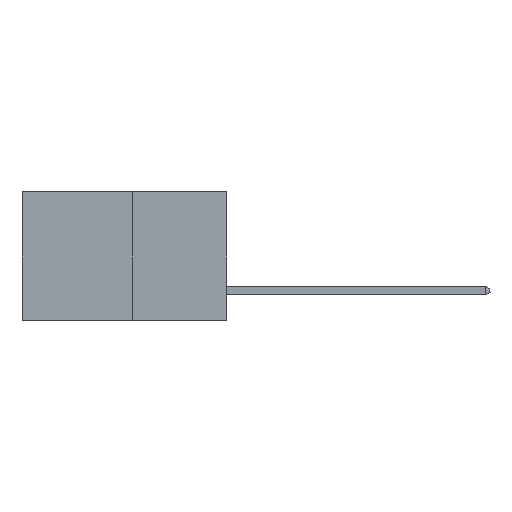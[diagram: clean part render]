
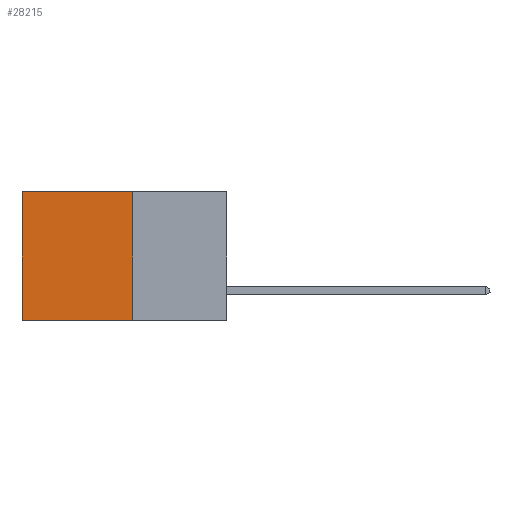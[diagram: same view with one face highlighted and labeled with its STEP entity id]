
A CAD part, left-side view. The second image highlights one B-rep face of the part: STEP entity #28215.
In plain terms, the highlighted planar face has unit normal (-1, 0, 0).
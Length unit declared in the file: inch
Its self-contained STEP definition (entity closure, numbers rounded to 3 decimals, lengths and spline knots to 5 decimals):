
#1632 = DIRECTION ( 'NONE',  ( 0., 0., -1. ) ) ;
#1753 = CARTESIAN_POINT ( 'NONE',  ( 0.277, 0.27, -0.37 ) ) ;
#2047 = AXIS2_PLACEMENT_3D ( 'NONE', #32463, #16976, #1632 ) ;
#2958 = ORIENTED_EDGE ( 'NONE', *, *, #8864, .T. ) ;
#3737 = FACE_OUTER_BOUND ( 'NONE', #17439, .T. ) ;
#4024 = VERTEX_POINT ( 'NONE', #24812 ) ;
#4605 = DIRECTION ( 'NONE',  ( 0., 1., 0. ) ) ;
#6934 = DIRECTION ( 'NONE',  ( 0., 0., -1. ) ) ;
#8864 = EDGE_CURVE ( 'NONE', #4024, #20282, #24092, .T. ) ;
#10590 = VECTOR ( 'NONE', #4605, 39.37008 ) ;
#11789 = EDGE_CURVE ( 'NONE', #11993, #17563, #14049, .T. ) ;
#11973 = ORIENTED_EDGE ( 'NONE', *, *, #11789, .F. ) ;
#11993 = VERTEX_POINT ( 'NONE', #14592 ) ;
#12102 = CARTESIAN_POINT ( 'NONE',  ( 0.277, 0.59, 0. ) ) ;
#12774 = LINE ( 'NONE', #1753, #32457 ) ;
#14049 = LINE ( 'NONE', #16102, #20712 ) ;
#14476 = PLANE ( 'NONE',  #2047 ) ;
#14592 = CARTESIAN_POINT ( 'NONE',  ( 0.277, 0.27, -0.37 ) ) ;
#16102 = CARTESIAN_POINT ( 'NONE',  ( 0.277, 0.27, -0.37 ) ) ;
#16832 = CARTESIAN_POINT ( 'NONE',  ( 0.277, 0.27, 0. ) ) ;
#16976 = DIRECTION ( 'NONE',  ( 1., 0., 0. ) ) ;
#17101 = VECTOR ( 'NONE', #32698, 39.37008 ) ;
#17185 = EDGE_CURVE ( 'NONE', #20282, #17563, #24667, .T. ) ;
#17186 = CARTESIAN_POINT ( 'NONE',  ( 0.277, 0.59, -0.37 ) ) ;
#17439 = EDGE_LOOP ( 'NONE', ( #31717, #11973, #23596, #2958 ) ) ;
#17563 = VERTEX_POINT ( 'NONE', #29127 ) ;
#20282 = VERTEX_POINT ( 'NONE', #12102 ) ;
#20712 = VECTOR ( 'NONE', #30758, 39.37008 ) ;
#23596 = ORIENTED_EDGE ( 'NONE', *, *, #25518, .F. ) ;
#24092 = LINE ( 'NONE', #16832, #10590 ) ;
#24667 = LINE ( 'NONE', #17186, #17101 ) ;
#24812 = CARTESIAN_POINT ( 'NONE',  ( 0.277, 0.27, 0. ) ) ;
#25518 = EDGE_CURVE ( 'NONE', #4024, #11993, #12774, .T. ) ;
#28215 = ADVANCED_FACE ( 'NONE', ( #3737 ), #14476, .F. ) ;
#29127 = CARTESIAN_POINT ( 'NONE',  ( 0.277, 0.59, -0.37 ) ) ;
#30758 = DIRECTION ( 'NONE',  ( 0., 1., 0. ) ) ;
#31717 = ORIENTED_EDGE ( 'NONE', *, *, #17185, .T. ) ;
#32457 = VECTOR ( 'NONE', #6934, 39.37008 ) ;
#32463 = CARTESIAN_POINT ( 'NONE',  ( 0.277, 0.27, -0.37 ) ) ;
#32698 = DIRECTION ( 'NONE',  ( 0., 0., -1. ) ) ;
